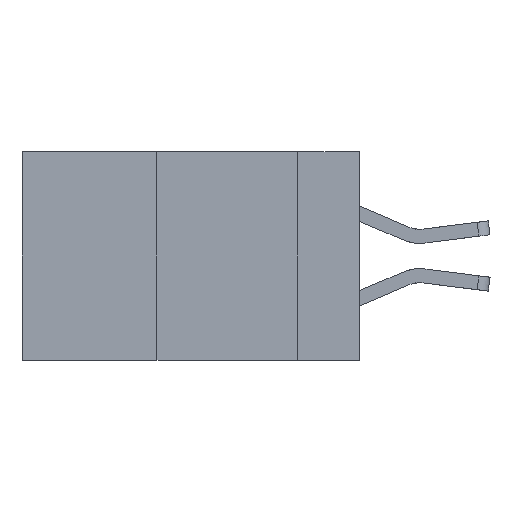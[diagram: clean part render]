
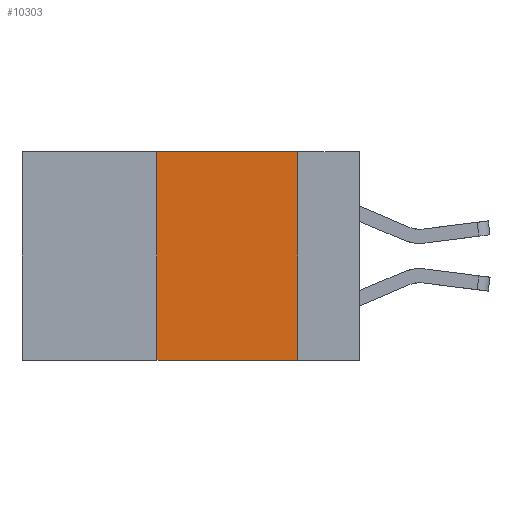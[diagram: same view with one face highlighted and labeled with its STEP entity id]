
A CAD part, left-side view. The second image highlights one B-rep face of the part: STEP entity #10303.
In plain terms, the highlighted planar face has unit normal (-1, 0, 0).
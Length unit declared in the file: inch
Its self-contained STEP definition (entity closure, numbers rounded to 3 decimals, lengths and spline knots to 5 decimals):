
#525 = EDGE_CURVE ( 'NONE', #8009, #715, #7920, .T. ) ;
#641 = DIRECTION ( 'NONE',  ( 0., -1., 0. ) ) ;
#703 = VECTOR ( 'NONE', #13523, 39.37008 ) ;
#715 = VERTEX_POINT ( 'NONE', #11504 ) ;
#921 = EDGE_LOOP ( 'NONE', ( #2938, #10173, #10112, #4376 ) ) ;
#1118 = CARTESIAN_POINT ( 'NONE',  ( 0., 0.11, 0. ) ) ;
#1133 = EDGE_CURVE ( 'NONE', #8009, #4535, #11540, .T. ) ;
#1663 = DIRECTION ( 'NONE',  ( 0., 0., -1. ) ) ;
#1719 = EDGE_CURVE ( 'NONE', #715, #5533, #12023, .T. ) ;
#2204 = DIRECTION ( 'NONE',  ( 0., 0., -1. ) ) ;
#2938 = ORIENTED_EDGE ( 'NONE', *, *, #7655, .F. ) ;
#3870 = CARTESIAN_POINT ( 'NONE',  ( 0., 0.36, 0. ) ) ;
#4376 = ORIENTED_EDGE ( 'NONE', *, *, #1133, .T. ) ;
#4535 = VERTEX_POINT ( 'NONE', #11133 ) ;
#5533 = VERTEX_POINT ( 'NONE', #12155 ) ;
#5755 = FACE_OUTER_BOUND ( 'NONE', #921, .T. ) ;
#6670 = VECTOR ( 'NONE', #2204, 39.37008 ) ;
#7403 = DIRECTION ( 'NONE',  ( 0., -1., 0. ) ) ;
#7655 = EDGE_CURVE ( 'NONE', #5533, #4535, #10637, .T. ) ;
#7920 = LINE ( 'NONE', #3870, #703 ) ;
#7974 = AXIS2_PLACEMENT_3D ( 'NONE', #8172, #11169, #1663 ) ;
#8009 = VERTEX_POINT ( 'NONE', #13346 ) ;
#8172 = CARTESIAN_POINT ( 'NONE',  ( 0., 0.6, 0. ) ) ;
#10112 = ORIENTED_EDGE ( 'NONE', *, *, #525, .F. ) ;
#10173 = ORIENTED_EDGE ( 'NONE', *, *, #1719, .F. ) ;
#10192 = CARTESIAN_POINT ( 'NONE',  ( 0., 0.6, -0.37 ) ) ;
#10303 = ADVANCED_FACE ( 'NONE', ( #5755 ), #11839, .F. ) ;
#10637 = LINE ( 'NONE', #1118, #6670 ) ;
#11133 = CARTESIAN_POINT ( 'NONE',  ( 0., 0.11, -0.37 ) ) ;
#11169 = DIRECTION ( 'NONE',  ( 1., 0., 0. ) ) ;
#11369 = VECTOR ( 'NONE', #641, 39.37008 ) ;
#11504 = CARTESIAN_POINT ( 'NONE',  ( 0., 0.36, 0. ) ) ;
#11540 = LINE ( 'NONE', #10192, #11369 ) ;
#11839 = PLANE ( 'NONE',  #7974 ) ;
#12023 = LINE ( 'NONE', #13719, #13019 ) ;
#12155 = CARTESIAN_POINT ( 'NONE',  ( 0., 0.11, 0. ) ) ;
#13019 = VECTOR ( 'NONE', #7403, 39.37008 ) ;
#13346 = CARTESIAN_POINT ( 'NONE',  ( 0., 0.36, -0.37 ) ) ;
#13523 = DIRECTION ( 'NONE',  ( 0., 0., 1. ) ) ;
#13719 = CARTESIAN_POINT ( 'NONE',  ( 0., 0.6, 0. ) ) ;
